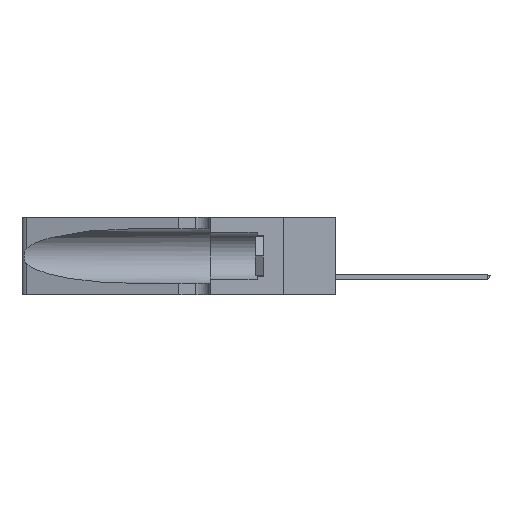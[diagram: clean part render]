
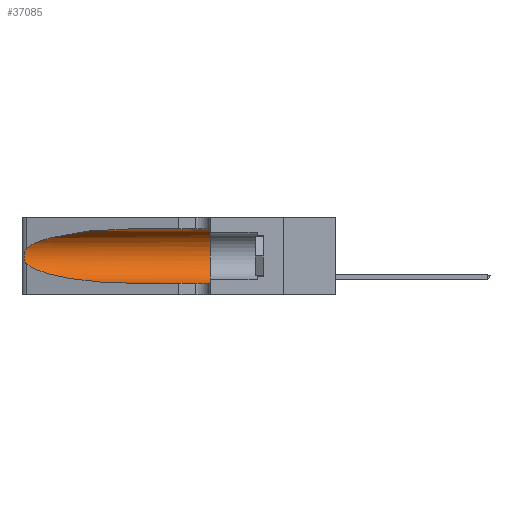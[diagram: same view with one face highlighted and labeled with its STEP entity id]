
A CAD part, left-side view. The second image highlights one B-rep face of the part: STEP entity #37085.
In plain terms, the highlighted cylindrical face has radius 3.308 mm (diameter 6.617 mm), a partial arc.
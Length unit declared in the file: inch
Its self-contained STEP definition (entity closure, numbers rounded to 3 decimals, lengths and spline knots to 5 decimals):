
#451 = CARTESIAN_POINT ( 'NONE',  ( 0.26017, 1.23833, 0.17102 ) ) ;
#596 = CARTESIAN_POINT ( 'NONE',  ( 0.25854, 1.2359, 0.20912 ) ) ;
#1114 = CYLINDRICAL_SURFACE ( 'NONE', #13962, 0.13025 ) ;
#1239 = CARTESIAN_POINT ( 'NONE',  ( 0.1305, 0.35, 0.05475 ) ) ;
#1297 = CARTESIAN_POINT ( 'NONE',  ( 0.1305, 0.35, 0.31525 ) ) ;
#1405 = CARTESIAN_POINT ( 'NONE',  ( 0.18966, 0.96281, 0.05475 ) ) ;
#2872 = CARTESIAN_POINT ( 'NONE',  ( 0.2373, 1.15595, 0.28018 ) ) ;
#3023 = CARTESIAN_POINT ( 'NONE',  ( 0.18966, 0.96281, 0.31525 ) ) ;
#3807 = EDGE_CURVE ( 'NONE', #16828, #29801, #15006, .T. ) ;
#4206 = CARTESIAN_POINT ( 'NONE',  ( 0.26018, 1.23835, 0.19895 ) ) ;
#4993 = CARTESIAN_POINT ( 'NONE',  ( 0.1305, 0.72297, 0.05475 ) ) ;
#6327 = DIRECTION ( 'NONE',  ( 0., 1., 0. ) ) ;
#7438 = ORIENTED_EDGE ( 'NONE', *, *, #16332, .T. ) ;
#7752 = CARTESIAN_POINT ( 'NONE',  ( 0.26075, 1.23896, 0.178 ) ) ;
#8055 = CARTESIAN_POINT ( 'NONE',  ( 0.25856, 1.23593, 0.16098 ) ) ;
#8342 = DIRECTION ( 'NONE',  ( 0., 0., -1. ) ) ;
#9437 = AXIS2_PLACEMENT_3D ( 'NONE', #37830, #6327, #38001 ) ;
#10228 = VERTEX_POINT ( 'NONE', #34544 ) ;
#11000 = CARTESIAN_POINT ( 'NONE',  ( 0.25787, 1.23484, 0.2124 ) ) ;
#12089 = CARTESIAN_POINT ( 'NONE',  ( 0.25487, 1.22718, 0.14631 ) ) ;
#13189 = DIRECTION ( 'NONE',  ( 0., -1., 0. ) ) ;
#13962 = AXIS2_PLACEMENT_3D ( 'NONE', #18601, #25880, #8342 ) ;
#14347 =( BOUNDED_CURVE ( )  B_SPLINE_CURVE ( 3, ( #12089, #43959, #1405, #4993 ),
 .UNSPECIFIED., .F., .F. ) 
 B_SPLINE_CURVE_WITH_KNOTS ( ( 4, 4 ),
 ( 3.44316, 4.71239 ),
 .UNSPECIFIED. ) 
 CURVE ( )  GEOMETRIC_REPRESENTATION_ITEM ( )  RATIONAL_B_SPLINE_CURVE ( ( 1., 0.87, 0.87, 1. ) ) 
 REPRESENTATION_ITEM ( '' )  );
#15006 = LINE ( 'NONE', #34164, #21681 ) ;
#15191 = CARTESIAN_POINT ( 'NONE',  ( 0.1305, 0.72297, 0.05475 ) ) ;
#15519 = EDGE_CURVE ( 'NONE', #10228, #45757, #22558, .T. ) ;
#16332 = EDGE_CURVE ( 'NONE', #17637, #16828, #14347, .T. ) ;
#16828 = VERTEX_POINT ( 'NONE', #15191 ) ;
#17553 = EDGE_LOOP ( 'NONE', ( #27984, #35130, #7438, #45012, #30860, #19249 ) ) ;
#17637 = VERTEX_POINT ( 'NONE', #41188 ) ;
#18162 = CARTESIAN_POINT ( 'NONE',  ( 0.25555, 1.22994, 0.2215 ) ) ;
#18601 = CARTESIAN_POINT ( 'NONE',  ( 0.1305, 1.61858, 0.185 ) ) ;
#19249 = ORIENTED_EDGE ( 'NONE', *, *, #42277, .F. ) ;
#21681 = VECTOR ( 'NONE', #13189, 39.37008 ) ;
#21724 = LINE ( 'NONE', #43202, #45159 ) ;
#22017 = CARTESIAN_POINT ( 'NONE',  ( 0.25789, 1.23486, 0.15765 ) ) ;
#22446 = EDGE_CURVE ( 'NONE', #36625, #29801, #41414, .T. ) ;
#22558 =( BOUNDED_CURVE ( )  B_SPLINE_CURVE ( 3, ( #38097, #3023, #2872, #45688 ),
 .UNSPECIFIED., .F., .F. ) 
 B_SPLINE_CURVE_WITH_KNOTS ( ( 4, 4 ),
 ( 1.5708, 2.84003 ),
 .UNSPECIFIED. ) 
 CURVE ( )  GEOMETRIC_REPRESENTATION_ITEM ( )  RATIONAL_B_SPLINE_CURVE ( ( 1., 0.87, 0.87, 1. ) ) 
 REPRESENTATION_ITEM ( '' )  );
#25429 = CARTESIAN_POINT ( 'NONE',  ( 0.25487, 1.22718, 0.14631 ) ) ;
#25880 = DIRECTION ( 'NONE',  ( 0., -1., 0. ) ) ;
#27984 = ORIENTED_EDGE ( 'NONE', *, *, #15519, .T. ) ;
#29341 = CARTESIAN_POINT ( 'NONE',  ( 0.26075, 1.23896, 0.19203 ) ) ;
#29801 = VERTEX_POINT ( 'NONE', #1239 ) ;
#30860 = ORIENTED_EDGE ( 'NONE', *, *, #22446, .F. ) ;
#32446 = CARTESIAN_POINT ( 'NONE',  ( 0.25555, 1.22993, 0.14849 ) ) ;
#34164 = CARTESIAN_POINT ( 'NONE',  ( 0.1305, 1.61858, 0.05475 ) ) ;
#34544 = CARTESIAN_POINT ( 'NONE',  ( 0.1305, 0.72297, 0.31525 ) ) ;
#35130 = ORIENTED_EDGE ( 'NONE', *, *, #45342, .T. ) ;
#35730 = CARTESIAN_POINT ( 'NONE',  ( 0.25639, 1.23186, 0.15144 ) ) ;
#36323 = CARTESIAN_POINT ( 'NONE',  ( 0.25639, 1.23184, 0.21858 ) ) ;
#36625 = VERTEX_POINT ( 'NONE', #1297 ) ;
#37085 = ADVANCED_FACE ( 'NONE', ( #38940 ), #1114, .F. ) ;
#37830 = CARTESIAN_POINT ( 'NONE',  ( 0.1305, 0.35, 0.185 ) ) ;
#38001 = DIRECTION ( 'NONE',  ( 0., 0., 1. ) ) ;
#38097 = CARTESIAN_POINT ( 'NONE',  ( 0.1305, 0.72297, 0.31525 ) ) ;
#38940 = FACE_OUTER_BOUND ( 'NONE', #17553, .T. ) ;
#40090 = DIRECTION ( 'NONE',  ( 0., -1., 0. ) ) ;
#41188 = CARTESIAN_POINT ( 'NONE',  ( 0.25487, 1.22718, 0.14631 ) ) ;
#41414 = CIRCLE ( 'NONE', #9437, 0.13025 ) ;
#42277 = EDGE_CURVE ( 'NONE', #10228, #36625, #21724, .T. ) ;
#43159 = CARTESIAN_POINT ( 'NONE',  ( 0.25487, 1.22718, 0.22369 ) ) ;
#43202 = CARTESIAN_POINT ( 'NONE',  ( 0.1305, 1.61858, 0.31525 ) ) ;
#43959 = CARTESIAN_POINT ( 'NONE',  ( 0.2373, 1.15595, 0.08982 ) ) ;
#45012 = ORIENTED_EDGE ( 'NONE', *, *, #3807, .T. ) ;
#45159 = VECTOR ( 'NONE', #40090, 39.37008 ) ;
#45342 = EDGE_CURVE ( 'NONE', #45757, #17637, #45398, .T. ) ;
#45361 = CARTESIAN_POINT ( 'NONE',  ( 0.25487, 1.22718, 0.22369 ) ) ;
#45398 = B_SPLINE_CURVE_WITH_KNOTS ( 'NONE', 3,
 ( #43159, #18162, #36323, #11000, #596, #4206, #29341, #7752, #451, #8055, #22017, #35730, #32446, #25429 ),
 .UNSPECIFIED., .F., .F.,
 ( 4, 2, 2, 2, 2, 2, 4 ),
 ( 0., 0.00027, 0.00053, 0.00107, 0.0016, 0.00187, 0.00214 ),
 .UNSPECIFIED. ) ;
#45688 = CARTESIAN_POINT ( 'NONE',  ( 0.25487, 1.22718, 0.22369 ) ) ;
#45757 = VERTEX_POINT ( 'NONE', #45361 ) ;
